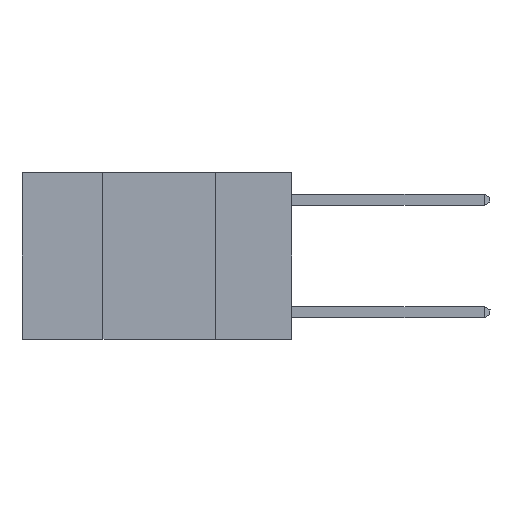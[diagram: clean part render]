
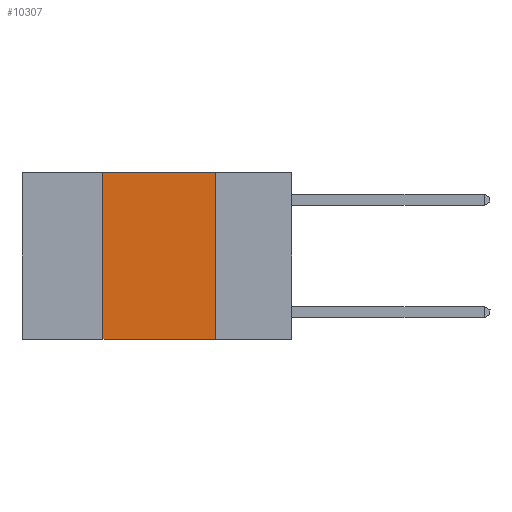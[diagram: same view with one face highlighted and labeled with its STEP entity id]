
A CAD part, left-side view. The second image highlights one B-rep face of the part: STEP entity #10307.
In plain terms, the highlighted planar face has unit normal (-1, 0, 0).
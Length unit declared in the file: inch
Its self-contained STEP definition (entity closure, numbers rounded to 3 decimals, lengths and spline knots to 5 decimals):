
#188 = ORIENTED_EDGE ( 'NONE', *, *, #12931, .F. ) ;
#215 = DIRECTION ( 'NONE',  ( 0., 0., -1. ) ) ;
#410 = DIRECTION ( 'NONE',  ( 0., -1., 0. ) ) ;
#518 = ORIENTED_EDGE ( 'NONE', *, *, #11248, .T. ) ;
#624 = VECTOR ( 'NONE', #215, 39.37008 ) ;
#1115 = VECTOR ( 'NONE', #410, 39.37008 ) ;
#1142 = DIRECTION ( 'NONE',  ( 0., 0., -1. ) ) ;
#1449 = LINE ( 'NONE', #2778, #1115 ) ;
#1727 = EDGE_CURVE ( 'NONE', #8396, #9945, #1449, .T. ) ;
#2277 = CARTESIAN_POINT ( 'NONE',  ( 0., 0.17, 0. ) ) ;
#2434 = VECTOR ( 'NONE', #5312, 39.37008 ) ;
#2778 = CARTESIAN_POINT ( 'NONE',  ( 0., 0.6, 0. ) ) ;
#3362 = CARTESIAN_POINT ( 'NONE',  ( 0., 0.42, -0.37 ) ) ;
#3610 = CARTESIAN_POINT ( 'NONE',  ( 0., 0.17, -0.37 ) ) ;
#3698 = CARTESIAN_POINT ( 'NONE',  ( 0., 0.17, 0. ) ) ;
#3891 = VECTOR ( 'NONE', #11710, 39.37008 ) ;
#5312 = DIRECTION ( 'NONE',  ( 0., 0., 1. ) ) ;
#5524 = LINE ( 'NONE', #2277, #624 ) ;
#5734 = CARTESIAN_POINT ( 'NONE',  ( 0., 0.6, -0.37 ) ) ;
#6231 = VERTEX_POINT ( 'NONE', #3362 ) ;
#6284 = ORIENTED_EDGE ( 'NONE', *, *, #11595, .F. ) ;
#7242 = CARTESIAN_POINT ( 'NONE',  ( 0., 0.6, 0. ) ) ;
#7283 = DIRECTION ( 'NONE',  ( 1., 0., 0. ) ) ;
#7577 = AXIS2_PLACEMENT_3D ( 'NONE', #7242, #7283, #1142 ) ;
#7592 = EDGE_LOOP ( 'NONE', ( #188, #11265, #6284, #518 ) ) ;
#8396 = VERTEX_POINT ( 'NONE', #12017 ) ;
#9240 = LINE ( 'NONE', #5734, #3891 ) ;
#9945 = VERTEX_POINT ( 'NONE', #3698 ) ;
#10307 = ADVANCED_FACE ( 'NONE', ( #10533 ), #11243, .F. ) ;
#10533 = FACE_OUTER_BOUND ( 'NONE', #7592, .T. ) ;
#11243 = PLANE ( 'NONE',  #7577 ) ;
#11248 = EDGE_CURVE ( 'NONE', #6231, #11824, #9240, .T. ) ;
#11265 = ORIENTED_EDGE ( 'NONE', *, *, #1727, .F. ) ;
#11300 = CARTESIAN_POINT ( 'NONE',  ( 0., 0.42, 0. ) ) ;
#11595 = EDGE_CURVE ( 'NONE', #6231, #8396, #12822, .T. ) ;
#11710 = DIRECTION ( 'NONE',  ( 0., -1., 0. ) ) ;
#11824 = VERTEX_POINT ( 'NONE', #3610 ) ;
#12017 = CARTESIAN_POINT ( 'NONE',  ( 0., 0.42, 0. ) ) ;
#12822 = LINE ( 'NONE', #11300, #2434 ) ;
#12931 = EDGE_CURVE ( 'NONE', #9945, #11824, #5524, .T. ) ;
